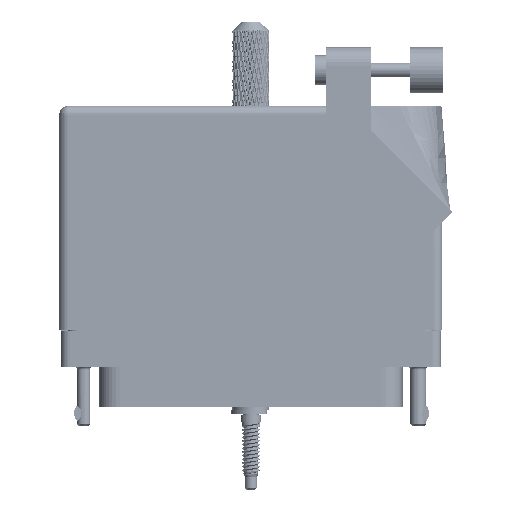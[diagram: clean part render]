
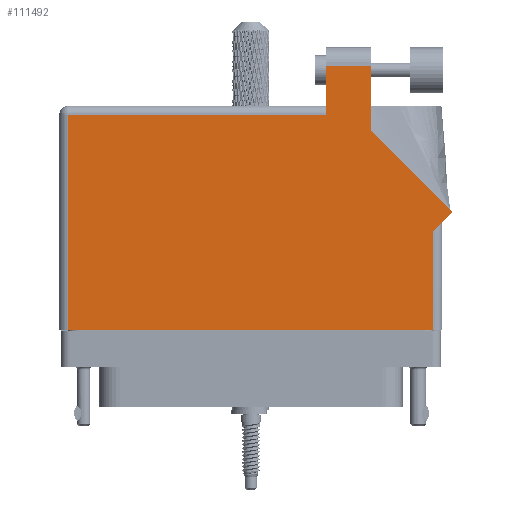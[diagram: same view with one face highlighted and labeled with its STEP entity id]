
A CAD part, front view. The second image highlights one B-rep face of the part: STEP entity #111492.
In plain terms, the highlighted face is planar.
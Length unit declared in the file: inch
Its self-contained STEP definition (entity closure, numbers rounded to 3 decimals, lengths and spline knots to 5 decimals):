
#9733 = VERTEX_POINT ( 'NONE', #121829 ) ;
#9774 = EDGE_CURVE ( 'NONE', #95543, #39203, #94714, .T. ) ;
#14222 = CARTESIAN_POINT ( 'NONE',  ( 0.513, 1.368, 0.455 ) ) ;
#16549 = CARTESIAN_POINT ( 'NONE',  ( -1.306, -0.1, 0.455 ) ) ;
#16921 = EDGE_CURVE ( 'NONE', #26226, #9733, #113972, .T. ) ;
#17285 = DIRECTION ( 'NONE',  ( -1., 0., 0. ) ) ;
#18046 = VECTOR ( 'NONE', #54601, 39.37008 ) ;
#18160 = CARTESIAN_POINT ( 'NONE',  ( 0.513, 1.705, 0.455 ) ) ;
#18249 = ORIENTED_EDGE ( 'NONE', *, *, #106657, .T. ) ;
#18653 = DIRECTION ( 'NONE',  ( -1., 0., 0. ) ) ;
#20314 = DIRECTION ( 'NONE',  ( 0., 1., 0. ) ) ;
#20660 = VERTEX_POINT ( 'NONE', #75917 ) ;
#21541 = DIRECTION ( 'NONE',  ( 0., 1., 0. ) ) ;
#21708 = ORIENTED_EDGE ( 'NONE', *, *, #40329, .T. ) ;
#23538 = EDGE_CURVE ( 'NONE', #38418, #113683, #91705, .T. ) ;
#26226 = VERTEX_POINT ( 'NONE', #68900 ) ;
#29793 = DIRECTION ( 'NONE',  ( -1., 0., 0. ) ) ;
#30843 = CARTESIAN_POINT ( 'NONE',  ( 1.37671, 0.70771, 0.455 ) ) ;
#33564 = EDGE_CURVE ( 'NONE', #20660, #76358, #51610, .T. ) ;
#33705 = ORIENTED_EDGE ( 'NONE', *, *, #110926, .T. ) ;
#38320 = CARTESIAN_POINT ( 'NONE',  ( -1.306, 1.43, 0.455 ) ) ;
#38418 = VERTEX_POINT ( 'NONE', #61669 ) ;
#39203 = VERTEX_POINT ( 'NONE', #14222 ) ;
#40329 = EDGE_CURVE ( 'NONE', #76358, #95543, #101795, .T. ) ;
#45862 = CARTESIAN_POINT ( 'NONE',  ( 0.82, 1.705, 0.455 ) ) ;
#48399 = LINE ( 'NONE', #115441, #71404 ) ;
#51390 = VECTOR ( 'NONE', #18653, 39.37008 ) ;
#51610 = LINE ( 'NONE', #60561, #94475 ) ;
#54601 = DIRECTION ( 'NONE',  ( 0., -1., 0. ) ) ;
#58024 = DIRECTION ( 'NONE',  ( 0., 0., -1. ) ) ;
#58516 = CARTESIAN_POINT ( 'NONE',  ( -1.306, 1.368, 0.455 ) ) ;
#58623 = VERTEX_POINT ( 'NONE', #30843 ) ;
#60050 = DIRECTION ( 'NONE',  ( -0.707, 0.707, 0. ) ) ;
#60561 = CARTESIAN_POINT ( 'NONE',  ( 0.82, 1.26442, 0.455 ) ) ;
#61011 = ORIENTED_EDGE ( 'NONE', *, *, #102598, .T. ) ;
#61669 = CARTESIAN_POINT ( 'NONE',  ( 1.244, -0.1, 0.455 ) ) ;
#66685 = DIRECTION ( 'NONE',  ( 0.707, 0.707, 0. ) ) ;
#67568 = VECTOR ( 'NONE', #103603, 39.37008 ) ;
#68900 = CARTESIAN_POINT ( 'NONE',  ( -1.244, 1.368, 0.455 ) ) ;
#71404 = VECTOR ( 'NONE', #66685, 39.37008 ) ;
#73853 = EDGE_LOOP ( 'NONE', ( #117829, #21708, #99423, #61011, #96514, #120061, #81515, #33705, #18249 ) ) ;
#75917 = CARTESIAN_POINT ( 'NONE',  ( 0.82, 1.26442, 0.455 ) ) ;
#75925 = LINE ( 'NONE', #58516, #51390 ) ;
#76358 = VERTEX_POINT ( 'NONE', #45862 ) ;
#76816 = VECTOR ( 'NONE', #60050, 39.37008 ) ;
#77457 = CARTESIAN_POINT ( 'NONE',  ( 0.513, 1.705, 0.455 ) ) ;
#78137 = CARTESIAN_POINT ( 'NONE',  ( 1.244, 0.637, 0.455 ) ) ;
#81515 = ORIENTED_EDGE ( 'NONE', *, *, #23538, .T. ) ;
#83447 = CARTESIAN_POINT ( 'NONE',  ( 1.244, 0.575, 0.455 ) ) ;
#85790 = CARTESIAN_POINT ( 'NONE',  ( -1.244, -0.1, 0.455 ) ) ;
#87988 = VECTOR ( 'NONE', #96095, 39.37008 ) ;
#91705 = LINE ( 'NONE', #78137, #119193 ) ;
#92595 = VECTOR ( 'NONE', #17285, 39.37008 ) ;
#94475 = VECTOR ( 'NONE', #21541, 39.37008 ) ;
#94714 = LINE ( 'NONE', #113225, #18046 ) ;
#95543 = VERTEX_POINT ( 'NONE', #77457 ) ;
#96095 = DIRECTION ( 'NONE',  ( 0., -1., 0. ) ) ;
#96514 = ORIENTED_EDGE ( 'NONE', *, *, #16921, .T. ) ;
#99423 = ORIENTED_EDGE ( 'NONE', *, *, #9774, .T. ) ;
#101795 = LINE ( 'NONE', #18160, #92595 ) ;
#102598 = EDGE_CURVE ( 'NONE', #39203, #26226, #75925, .T. ) ;
#103431 = AXIS2_PLACEMENT_3D ( 'NONE', #38320, #58024, #29793 ) ;
#103603 = DIRECTION ( 'NONE',  ( 1., 0., 0. ) ) ;
#104997 = FACE_OUTER_BOUND ( 'NONE', #73853, .T. ) ;
#106657 = EDGE_CURVE ( 'NONE', #58623, #20660, #122742, .T. ) ;
#110442 = LINE ( 'NONE', #16549, #67568 ) ;
#110926 = EDGE_CURVE ( 'NONE', #113683, #58623, #48399, .T. ) ;
#111492 = ADVANCED_FACE ( 'NONE', ( #104997 ), #118355, .F. ) ;
#113225 = CARTESIAN_POINT ( 'NONE',  ( 0.513, 1.43, 0.455 ) ) ;
#113683 = VERTEX_POINT ( 'NONE', #83447 ) ;
#113972 = LINE ( 'NONE', #85790, #87988 ) ;
#115079 = EDGE_CURVE ( 'NONE', #9733, #38418, #110442, .T. ) ;
#115441 = CARTESIAN_POINT ( 'NONE',  ( 1.306, 0.637, 0.455 ) ) ;
#117829 = ORIENTED_EDGE ( 'NONE', *, *, #33564, .T. ) ;
#118224 = CARTESIAN_POINT ( 'NONE',  ( 1.37671, 0.70771, 0.455 ) ) ;
#118355 = PLANE ( 'NONE',  #103431 ) ;
#119193 = VECTOR ( 'NONE', #20314, 39.37008 ) ;
#120061 = ORIENTED_EDGE ( 'NONE', *, *, #115079, .T. ) ;
#121829 = CARTESIAN_POINT ( 'NONE',  ( -1.244, -0.1, 0.455 ) ) ;
#122742 = LINE ( 'NONE', #118224, #76816 ) ;
